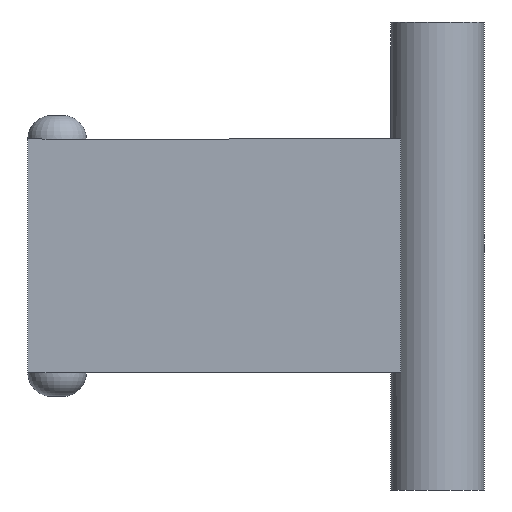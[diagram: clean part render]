
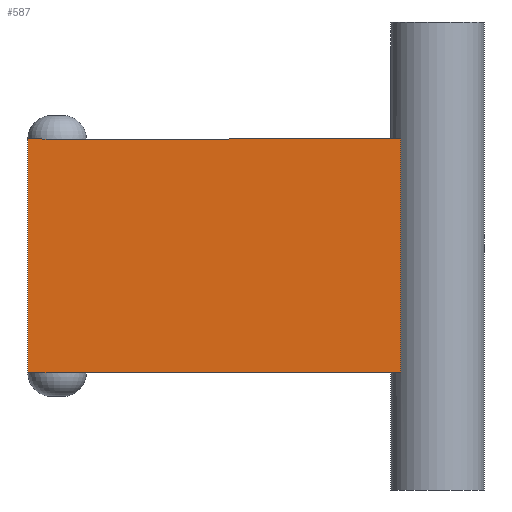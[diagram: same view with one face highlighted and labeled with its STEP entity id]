
A CAD part, front view. The second image highlights one B-rep face of the part: STEP entity #587.
In plain terms, the highlighted planar face has unit normal (0, -1, 0).
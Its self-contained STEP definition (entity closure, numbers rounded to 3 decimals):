
#12 = VERTEX_POINT ( 'NONE', #179 ) ;
#16 = VECTOR ( 'NONE', #506, 1000. ) ;
#34 = EDGE_CURVE ( 'NONE', #541, #269, #483, .T. ) ;
#77 = LINE ( 'NONE', #416, #212 ) ;
#90 = EDGE_CURVE ( 'NONE', #269, #253, #77, .T. ) ;
#91 = VECTOR ( 'NONE', #474, 1000. ) ;
#95 = VECTOR ( 'NONE', #449, 1000. ) ;
#105 = CARTESIAN_POINT ( 'NONE',  ( -17.5, 0., 10. ) ) ;
#109 = FACE_OUTER_BOUND ( 'NONE', #341, .T. ) ;
#114 = VERTEX_POINT ( 'NONE', #588 ) ;
#133 = CARTESIAN_POINT ( 'NONE',  ( -17.5, 0., 10. ) ) ;
#139 = VECTOR ( 'NONE', #263, 1000. ) ;
#156 = AXIS2_PLACEMENT_3D ( 'NONE', #227, #230, #563 ) ;
#179 = CARTESIAN_POINT ( 'NONE',  ( -15., 0., -10. ) ) ;
#181 = ORIENTED_EDGE ( 'NONE', *, *, #505, .F. ) ;
#200 = EDGE_CURVE ( 'NONE', #114, #255, #258, .T. ) ;
#204 = VECTOR ( 'NONE', #412, 1000. ) ;
#212 = VECTOR ( 'NONE', #421, 1000. ) ;
#227 = CARTESIAN_POINT ( 'NONE',  ( 0., 0., 0. ) ) ;
#230 = DIRECTION ( 'NONE',  ( 0., -1., 0. ) ) ;
#253 = VERTEX_POINT ( 'NONE', #377 ) ;
#255 = VERTEX_POINT ( 'NONE', #613 ) ;
#258 = LINE ( 'NONE', #133, #139 ) ;
#263 = DIRECTION ( 'NONE',  ( 0., 0., 1. ) ) ;
#269 = VERTEX_POINT ( 'NONE', #371 ) ;
#285 = ORIENTED_EDGE ( 'NONE', *, *, #34, .F. ) ;
#323 = EDGE_CURVE ( 'NONE', #12, #114, #340, .T. ) ;
#333 = ORIENTED_EDGE ( 'NONE', *, *, #350, .F. ) ;
#340 = LINE ( 'NONE', #454, #95 ) ;
#341 = EDGE_LOOP ( 'NONE', ( #285, #333, #572, #440, #181, #548 ) ) ;
#350 = EDGE_CURVE ( 'NONE', #255, #541, #570, .T. ) ;
#360 = CARTESIAN_POINT ( 'NONE',  ( -17.5, 0., -10. ) ) ;
#371 = CARTESIAN_POINT ( 'NONE',  ( 14.378, 0., 10. ) ) ;
#377 = CARTESIAN_POINT ( 'NONE',  ( 14.378, 0., -10. ) ) ;
#412 = DIRECTION ( 'NONE',  ( 1., 0., 0. ) ) ;
#416 = CARTESIAN_POINT ( 'NONE',  ( 14.378, 0., -20. ) ) ;
#421 = DIRECTION ( 'NONE',  ( 0., 0., -1. ) ) ;
#422 = PLANE ( 'NONE',  #156 ) ;
#440 = ORIENTED_EDGE ( 'NONE', *, *, #323, .F. ) ;
#449 = DIRECTION ( 'NONE',  ( -1., 0., 0. ) ) ;
#454 = CARTESIAN_POINT ( 'NONE',  ( -17.5, 0., -10. ) ) ;
#464 = CARTESIAN_POINT ( 'NONE',  ( -15., 0., 10. ) ) ;
#467 = CARTESIAN_POINT ( 'NONE',  ( -17.5, 0., 10. ) ) ;
#474 = DIRECTION ( 'NONE',  ( 1., 0., 0. ) ) ;
#483 = LINE ( 'NONE', #105, #91 ) ;
#505 = EDGE_CURVE ( 'NONE', #253, #12, #527, .T. ) ;
#506 = DIRECTION ( 'NONE',  ( -1., 0., 0. ) ) ;
#527 = LINE ( 'NONE', #360, #16 ) ;
#541 = VERTEX_POINT ( 'NONE', #464 ) ;
#548 = ORIENTED_EDGE ( 'NONE', *, *, #90, .F. ) ;
#563 = DIRECTION ( 'NONE',  ( 0., 0., -1. ) ) ;
#570 = LINE ( 'NONE', #467, #204 ) ;
#572 = ORIENTED_EDGE ( 'NONE', *, *, #200, .F. ) ;
#587 = ADVANCED_FACE ( 'NONE', ( #109 ), #422, .T. ) ;
#588 = CARTESIAN_POINT ( 'NONE',  ( -17.5, 0., -10. ) ) ;
#613 = CARTESIAN_POINT ( 'NONE',  ( -17.5, 0., 10. ) ) ;
